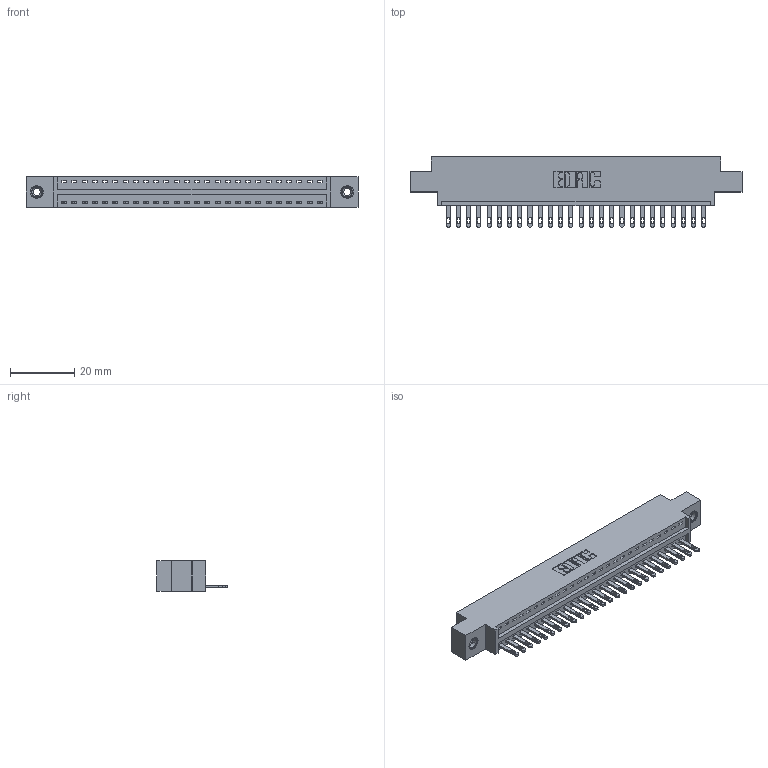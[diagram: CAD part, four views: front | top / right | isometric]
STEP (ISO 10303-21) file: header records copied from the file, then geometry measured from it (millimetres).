
FILE_DESCRIPTION (( 'STEP AP203' ), '1' );
FILE_NAME ('896-026-500-608.STEP', '2021-07-27T17:58:42', ( '' ), ( '' ), 'SwSTEP 2.0', 'SolidWorks 2020', '' );
FILE_SCHEMA (( 'CONFIG_CONTROL_DESIGN' ));
Length unit declared in the file: inch
Products named in the file (4): 345-250-001_345-250-003-102; 345-292-001_345-293-100; 846 Part_0.170 Offset - 0.156 Dia-TI; 896-026-500-608
Assembly tree (29 placements, depth 2):
  896-026-500-608
    846 Part_0.170 Offset - 0.156 Dia-TI
    345-292-001_345-293-100  x26
    345-250-001_345-250-003-102  x2
Bounding box: 103.12 x 21.84 x 9.4 mm (x, y, z)
Volume: 9616 mm3; surface area: 12088.8 mm2
Topology: 29 solids, 29 shells, 1590 faces, 4845 edges, 3222 vertices
Faces by surface type: plane 996, cylinder 578, cone 12, torus 4
Entity records: 19538 total; most frequent: CARTESIAN_POINT 3337, ORIENTED_EDGE 3290, DIRECTION 2991, EDGE_CURVE 1645, VECTOR 1385, LINE 1385, VERTEX_POINT 1092, AXIS2_PLACEMENT_3D 803
